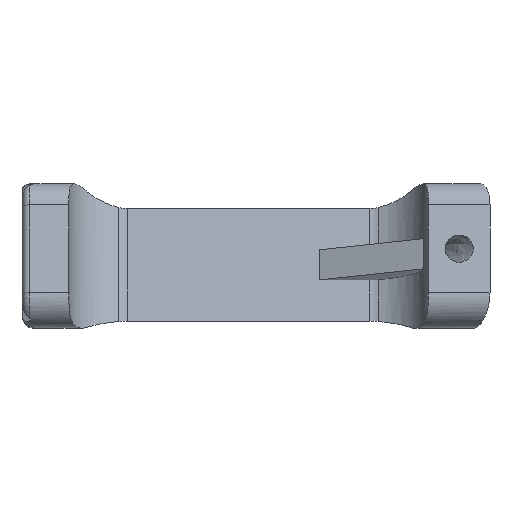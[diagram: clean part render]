
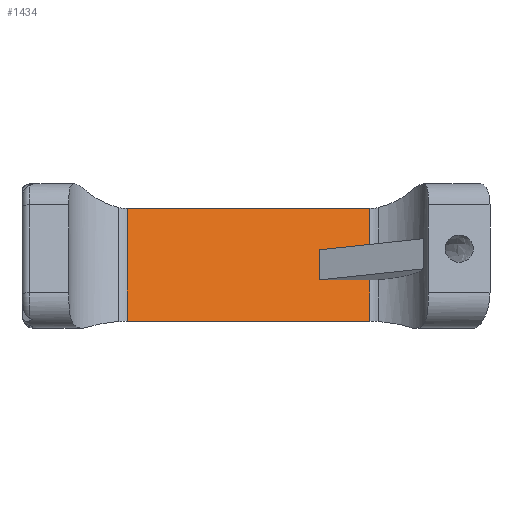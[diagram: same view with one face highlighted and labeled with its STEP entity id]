
A CAD part, front view. The second image highlights one B-rep face of the part: STEP entity #1434.
In plain terms, the highlighted planar face has unit normal (0, -0.966, 0.259).
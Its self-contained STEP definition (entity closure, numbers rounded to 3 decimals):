
#234=FACE_OUTER_BOUND('',#313,.T.);
#313=EDGE_LOOP('',(#1211,#1212,#1213,#1214,#1215,#1216,#1217,#1218));
#338=LINE('',#2028,#435);
#342=LINE('',#2080,#439);
#343=LINE('',#2085,#440);
#389=LINE('',#2903,#486);
#395=LINE('',#2936,#492);
#396=LINE('',#2937,#493);
#397=LINE('',#2939,#494);
#398=LINE('',#2940,#495);
#435=VECTOR('',#1625,10.);
#439=VECTOR('',#1641,10.);
#440=VECTOR('',#1648,10.);
#486=VECTOR('',#1918,10.);
#492=VECTOR('',#1938,10.);
#493=VECTOR('',#1939,10.);
#494=VECTOR('',#1940,10.);
#495=VECTOR('',#1941,10.);
#530=VERTEX_POINT('',#2022);
#532=VERTEX_POINT('',#2026);
#542=VERTEX_POINT('',#2079);
#543=VERTEX_POINT('',#2083);
#645=VERTEX_POINT('',#2899);
#646=VERTEX_POINT('',#2901);
#650=VERTEX_POINT('',#2935);
#651=VERTEX_POINT('',#2938);
#675=EDGE_CURVE('',#530,#532,#338,.T.);
#686=EDGE_CURVE('',#542,#530,#342,.T.);
#689=EDGE_CURVE('',#532,#543,#343,.T.);
#841=EDGE_CURVE('',#646,#645,#389,.T.);
#850=EDGE_CURVE('',#650,#646,#395,.T.);
#851=EDGE_CURVE('',#542,#650,#396,.T.);
#852=EDGE_CURVE('',#651,#543,#397,.T.);
#853=EDGE_CURVE('',#645,#651,#398,.T.);
#1211=ORIENTED_EDGE('',*,*,#850,.F.);
#1212=ORIENTED_EDGE('',*,*,#851,.F.);
#1213=ORIENTED_EDGE('',*,*,#686,.T.);
#1214=ORIENTED_EDGE('',*,*,#675,.T.);
#1215=ORIENTED_EDGE('',*,*,#689,.T.);
#1216=ORIENTED_EDGE('',*,*,#852,.F.);
#1217=ORIENTED_EDGE('',*,*,#853,.F.);
#1218=ORIENTED_EDGE('',*,*,#841,.F.);
#1359=PLANE('',#1595);
#1434=ADVANCED_FACE('',(#234),#1359,.F.);
#1595=AXIS2_PLACEMENT_3D('',#2934,#1936,#1937);
#1625=DIRECTION('',(0.,0.259,0.966));
#1641=DIRECTION('',(-1.,0.,0.));
#1648=DIRECTION('',(1.,0.,0.));
#1918=DIRECTION('',(0.,0.259,0.966));
#1936=DIRECTION('center_axis',(0.,0.966,-0.259));
#1937=DIRECTION('ref_axis',(1.,0.,0.));
#1938=DIRECTION('',(-1.,0.,0.));
#1939=DIRECTION('',(0.,-0.259,-0.966));
#1940=DIRECTION('',(0.,-0.259,-0.966));
#1941=DIRECTION('',(1.,0.,0.));
#2022=CARTESIAN_POINT('',(-12.35,32.247,-53.881));
#2026=CARTESIAN_POINT('',(-12.35,32.764,-51.949));
#2028=CARTESIAN_POINT('',(-12.35,32.635,-52.432));
#2079=CARTESIAN_POINT('',(-9.112,32.247,-53.881));
#2080=CARTESIAN_POINT('',(-18.612,32.247,-53.881));
#2083=CARTESIAN_POINT('',(-9.112,32.764,-51.949));
#2085=CARTESIAN_POINT('',(-15.112,32.764,-51.949));
#2899=CARTESIAN_POINT('',(-24.638,33.473,-49.304));
#2901=CARTESIAN_POINT('',(-24.638,31.538,-56.526));
#2903=CARTESIAN_POINT('',(-24.638,32.506,-52.915));
#2934=CARTESIAN_POINT('Origin',(-24.875,32.506,-52.915));
#2935=CARTESIAN_POINT('',(-9.112,31.538,-56.526));
#2936=CARTESIAN_POINT('',(-28.137,31.538,-56.526));
#2937=CARTESIAN_POINT('',(-9.112,32.506,-52.915));
#2938=CARTESIAN_POINT('',(-9.112,33.473,-49.304));
#2939=CARTESIAN_POINT('',(-9.112,32.506,-52.915));
#2940=CARTESIAN_POINT('',(-28.137,33.473,-49.304));
